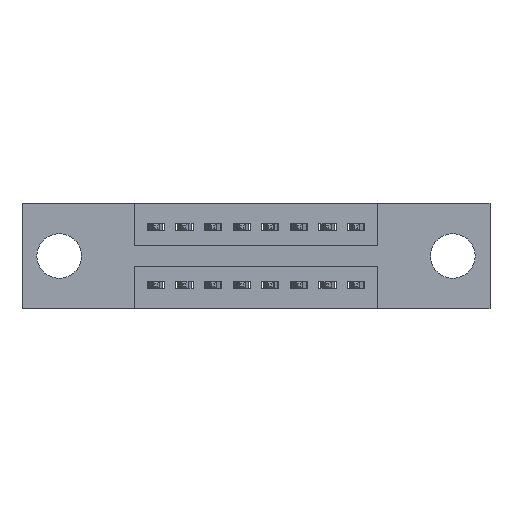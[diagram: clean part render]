
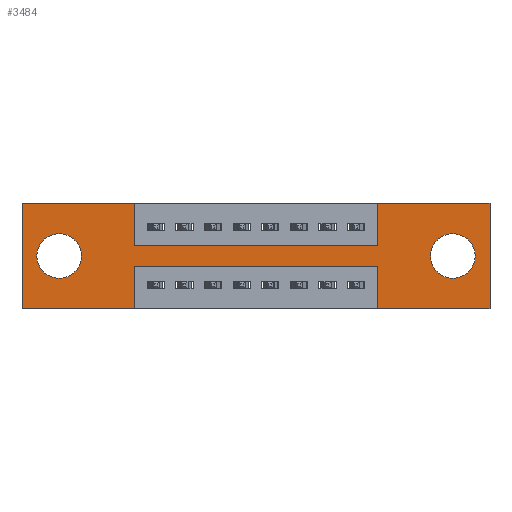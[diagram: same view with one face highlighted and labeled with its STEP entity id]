
A CAD part, front view. The second image highlights one B-rep face of the part: STEP entity #3484.
In plain terms, the highlighted planar face has unit normal (0, -1, 0).
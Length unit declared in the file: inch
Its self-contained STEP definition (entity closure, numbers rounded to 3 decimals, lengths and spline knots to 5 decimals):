
#56 = VERTEX_POINT ( 'NONE', #6474 ) ;
#128 = LINE ( 'NONE', #3564, #10887 ) ;
#141 = ORIENTED_EDGE ( 'NONE', *, *, #2143, .T. ) ;
#294 = CARTESIAN_POINT ( 'NONE',  ( 1.2425, 0., -0.37 ) ) ;
#381 = VERTEX_POINT ( 'NONE', #1865 ) ;
#614 = CARTESIAN_POINT ( 'NONE',  ( 0.13, 0., -0.185 ) ) ;
#624 = DIRECTION ( 'NONE',  ( 0., 1., 0. ) ) ;
#770 = ORIENTED_EDGE ( 'NONE', *, *, #3946, .T. ) ;
#771 = LINE ( 'NONE', #4481, #2104 ) ;
#1072 = VERTEX_POINT ( 'NONE', #7731 ) ;
#1081 = AXIS2_PLACEMENT_3D ( 'NONE', #614, #1631, #11090 ) ;
#1167 = PLANE ( 'NONE',  #10337 ) ;
#1365 = VECTOR ( 'NONE', #10003, 39.37008 ) ;
#1389 = ORIENTED_EDGE ( 'NONE', *, *, #3904, .T. ) ;
#1414 = ORIENTED_EDGE ( 'NONE', *, *, #4028, .F. ) ;
#1590 = DIRECTION ( 'NONE',  ( 0., 1., 0. ) ) ;
#1601 = VECTOR ( 'NONE', #9488, 39.37008 ) ;
#1631 = DIRECTION ( 'NONE',  ( 0., 1., 0. ) ) ;
#1865 = CARTESIAN_POINT ( 'NONE',  ( 0.3925, 0., -0.22 ) ) ;
#1912 = CIRCLE ( 'NONE', #9963, 0.078 ) ;
#2054 = EDGE_CURVE ( 'NONE', #2302, #4044, #771, .T. ) ;
#2103 = AXIS2_PLACEMENT_3D ( 'NONE', #3262, #624, #6704 ) ;
#2104 = VECTOR ( 'NONE', #9747, 39.37008 ) ;
#2143 = EDGE_CURVE ( 'NONE', #4229, #1072, #1912, .T. ) ;
#2271 = LINE ( 'NONE', #6739, #10328 ) ;
#2286 = VECTOR ( 'NONE', #9375, 39.37008 ) ;
#2302 = VERTEX_POINT ( 'NONE', #9396 ) ;
#2312 = VERTEX_POINT ( 'NONE', #2362 ) ;
#2362 = CARTESIAN_POINT ( 'NONE',  ( 1.2425, 0., -0.15 ) ) ;
#2506 = EDGE_CURVE ( 'NONE', #9969, #2302, #128, .T. ) ;
#2737 = EDGE_LOOP ( 'NONE', ( #770, #8006 ) ) ;
#2803 = DIRECTION ( 'NONE',  ( 0., 0., -1. ) ) ;
#2893 = DIRECTION ( 'NONE',  ( 0., 0., -1. ) ) ;
#2895 = CARTESIAN_POINT ( 'NONE',  ( 0., 0., -0.37 ) ) ;
#3186 = ORIENTED_EDGE ( 'NONE', *, *, #4300, .F. ) ;
#3262 = CARTESIAN_POINT ( 'NONE',  ( 1.505, 0., -0.185 ) ) ;
#3317 = LINE ( 'NONE', #9314, #1601 ) ;
#3342 = DIRECTION ( 'NONE',  ( 0., 0., 1. ) ) ;
#3469 = LINE ( 'NONE', #5194, #10599 ) ;
#3484 = ADVANCED_FACE ( 'NONE', ( #5645, #8948, #8096 ), #1167, .T. ) ;
#3541 = LINE ( 'NONE', #4501, #6205 ) ;
#3564 = CARTESIAN_POINT ( 'NONE',  ( 0., 0., 0. ) ) ;
#3904 = EDGE_CURVE ( 'NONE', #1072, #4229, #10319, .T. ) ;
#3946 = EDGE_CURVE ( 'NONE', #6277, #10006, #5950, .T. ) ;
#4001 = CARTESIAN_POINT ( 'NONE',  ( 0.3925, 0., -0.37 ) ) ;
#4028 = EDGE_CURVE ( 'NONE', #6402, #381, #8467, .T. ) ;
#4044 = VERTEX_POINT ( 'NONE', #5149 ) ;
#4045 = DIRECTION ( 'NONE',  ( 0., 0., 1. ) ) ;
#4150 = DIRECTION ( 'NONE',  ( 0., 0., -1. ) ) ;
#4229 = VERTEX_POINT ( 'NONE', #8909 ) ;
#4300 = EDGE_CURVE ( 'NONE', #4044, #2312, #5488, .T. ) ;
#4401 = CARTESIAN_POINT ( 'NONE',  ( 0., 0., 0. ) ) ;
#4447 = EDGE_CURVE ( 'NONE', #381, #7881, #2271, .T. ) ;
#4481 = CARTESIAN_POINT ( 'NONE',  ( 0.3925, 0., 0. ) ) ;
#4501 = CARTESIAN_POINT ( 'NONE',  ( 1.635, 0., 0. ) ) ;
#4542 = CARTESIAN_POINT ( 'NONE',  ( 0., 0., 0. ) ) ;
#4575 = EDGE_CURVE ( 'NONE', #9108, #10489, #7134, .T. ) ;
#4596 = DIRECTION ( 'NONE',  ( 0., 0., -1. ) ) ;
#4633 = DIRECTION ( 'NONE',  ( 0., 0., 1. ) ) ;
#4655 = CARTESIAN_POINT ( 'NONE',  ( 1.505, 0., -0.185 ) ) ;
#4678 = VERTEX_POINT ( 'NONE', #8953 ) ;
#4732 = EDGE_LOOP ( 'NONE', ( #6372, #1414, #6492, #9165, #5458, #6764, #5681, #3186, #6796, #7961, #10584, #8187 ) ) ;
#4871 = EDGE_CURVE ( 'NONE', #56, #9969, #5334, .T. ) ;
#5013 = EDGE_CURVE ( 'NONE', #2312, #9108, #8306, .T. ) ;
#5118 = CARTESIAN_POINT ( 'NONE',  ( 0.13, 0., -0.107 ) ) ;
#5149 = CARTESIAN_POINT ( 'NONE',  ( 0.3925, 0., -0.15 ) ) ;
#5194 = CARTESIAN_POINT ( 'NONE',  ( 0., 0., -0.37 ) ) ;
#5227 = DIRECTION ( 'NONE',  ( 1., 0., 0. ) ) ;
#5232 = EDGE_CURVE ( 'NONE', #7881, #56, #3317, .T. ) ;
#5244 = CARTESIAN_POINT ( 'NONE',  ( 0., 0., 0. ) ) ;
#5334 = LINE ( 'NONE', #4401, #10747 ) ;
#5394 = EDGE_CURVE ( 'NONE', #10489, #4678, #3541, .T. ) ;
#5458 = ORIENTED_EDGE ( 'NONE', *, *, #5394, .F. ) ;
#5488 = LINE ( 'NONE', #9948, #1365 ) ;
#5645 = FACE_BOUND ( 'NONE', #9256, .T. ) ;
#5681 = ORIENTED_EDGE ( 'NONE', *, *, #5013, .F. ) ;
#5902 = CARTESIAN_POINT ( 'NONE',  ( 0.3925, 0., -0.22 ) ) ;
#5950 = CIRCLE ( 'NONE', #10133, 0.078 ) ;
#6032 = CIRCLE ( 'NONE', #1081, 0.078 ) ;
#6205 = VECTOR ( 'NONE', #2803, 39.37008 ) ;
#6277 = VERTEX_POINT ( 'NONE', #5118 ) ;
#6372 = ORIENTED_EDGE ( 'NONE', *, *, #4447, .F. ) ;
#6402 = VERTEX_POINT ( 'NONE', #10714 ) ;
#6474 = CARTESIAN_POINT ( 'NONE',  ( 0., 0., -0.37 ) ) ;
#6492 = ORIENTED_EDGE ( 'NONE', *, *, #6970, .F. ) ;
#6595 = CARTESIAN_POINT ( 'NONE',  ( 1.2425, 0., 0. ) ) ;
#6691 = VECTOR ( 'NONE', #10438, 39.37008 ) ;
#6704 = DIRECTION ( 'NONE',  ( 0., 0., -1. ) ) ;
#6739 = CARTESIAN_POINT ( 'NONE',  ( 0.3925, 0., -0.37 ) ) ;
#6764 = ORIENTED_EDGE ( 'NONE', *, *, #4575, .F. ) ;
#6796 = ORIENTED_EDGE ( 'NONE', *, *, #2054, .F. ) ;
#6970 = EDGE_CURVE ( 'NONE', #9048, #6402, #10281, .T. ) ;
#7134 = LINE ( 'NONE', #5244, #6691 ) ;
#7465 = CARTESIAN_POINT ( 'NONE',  ( 1.635, 0., 0. ) ) ;
#7502 = CARTESIAN_POINT ( 'NONE',  ( 0.13, 0., -0.185 ) ) ;
#7731 = CARTESIAN_POINT ( 'NONE',  ( 1.505, 0., -0.107 ) ) ;
#7874 = DIRECTION ( 'NONE',  ( -1., 0., 0. ) ) ;
#7881 = VERTEX_POINT ( 'NONE', #4001 ) ;
#7961 = ORIENTED_EDGE ( 'NONE', *, *, #2506, .F. ) ;
#8006 = ORIENTED_EDGE ( 'NONE', *, *, #9620, .T. ) ;
#8096 = FACE_OUTER_BOUND ( 'NONE', #4732, .T. ) ;
#8106 = CARTESIAN_POINT ( 'NONE',  ( 0.13, 0., -0.263 ) ) ;
#8187 = ORIENTED_EDGE ( 'NONE', *, *, #5232, .F. ) ;
#8306 = LINE ( 'NONE', #9907, #8372 ) ;
#8372 = VECTOR ( 'NONE', #4633, 39.37008 ) ;
#8467 = LINE ( 'NONE', #5902, #2286 ) ;
#8909 = CARTESIAN_POINT ( 'NONE',  ( 1.505, 0., -0.263 ) ) ;
#8948 = FACE_BOUND ( 'NONE', #2737, .T. ) ;
#8953 = CARTESIAN_POINT ( 'NONE',  ( 1.635, 0., -0.37 ) ) ;
#9008 = DIRECTION ( 'NONE',  ( 0., -1., 0. ) ) ;
#9048 = VERTEX_POINT ( 'NONE', #294 ) ;
#9108 = VERTEX_POINT ( 'NONE', #6595 ) ;
#9141 = VECTOR ( 'NONE', #4045, 39.37008 ) ;
#9165 = ORIENTED_EDGE ( 'NONE', *, *, #9833, .F. ) ;
#9256 = EDGE_LOOP ( 'NONE', ( #1389, #141 ) ) ;
#9314 = CARTESIAN_POINT ( 'NONE',  ( 0., 0., -0.37 ) ) ;
#9375 = DIRECTION ( 'NONE',  ( -1., 0., 0. ) ) ;
#9396 = CARTESIAN_POINT ( 'NONE',  ( 0.3925, 0., 0. ) ) ;
#9423 = CARTESIAN_POINT ( 'NONE',  ( 1.2425, 0., -0.37 ) ) ;
#9488 = DIRECTION ( 'NONE',  ( -1., 0., 0. ) ) ;
#9620 = EDGE_CURVE ( 'NONE', #10006, #6277, #6032, .T. ) ;
#9747 = DIRECTION ( 'NONE',  ( 0., 0., -1. ) ) ;
#9833 = EDGE_CURVE ( 'NONE', #4678, #9048, #3469, .T. ) ;
#9907 = CARTESIAN_POINT ( 'NONE',  ( 1.2425, 0., 0. ) ) ;
#9948 = CARTESIAN_POINT ( 'NONE',  ( 0.3925, 0., -0.15 ) ) ;
#9963 = AXIS2_PLACEMENT_3D ( 'NONE', #4655, #10720, #2893 ) ;
#9969 = VERTEX_POINT ( 'NONE', #4542 ) ;
#10003 = DIRECTION ( 'NONE',  ( 1., 0., 0. ) ) ;
#10006 = VERTEX_POINT ( 'NONE', #8106 ) ;
#10133 = AXIS2_PLACEMENT_3D ( 'NONE', #7502, #1590, #10987 ) ;
#10281 = LINE ( 'NONE', #9423, #9141 ) ;
#10319 = CIRCLE ( 'NONE', #2103, 0.078 ) ;
#10328 = VECTOR ( 'NONE', #4150, 39.37008 ) ;
#10337 = AXIS2_PLACEMENT_3D ( 'NONE', #2895, #9008, #4596 ) ;
#10438 = DIRECTION ( 'NONE',  ( 1., 0., 0. ) ) ;
#10489 = VERTEX_POINT ( 'NONE', #7465 ) ;
#10584 = ORIENTED_EDGE ( 'NONE', *, *, #4871, .F. ) ;
#10599 = VECTOR ( 'NONE', #7874, 39.37008 ) ;
#10714 = CARTESIAN_POINT ( 'NONE',  ( 1.2425, 0., -0.22 ) ) ;
#10720 = DIRECTION ( 'NONE',  ( 0., 1., 0. ) ) ;
#10747 = VECTOR ( 'NONE', #3342, 39.37008 ) ;
#10887 = VECTOR ( 'NONE', #5227, 39.37008 ) ;
#10987 = DIRECTION ( 'NONE',  ( 0., 0., 1. ) ) ;
#11090 = DIRECTION ( 'NONE',  ( 0., 0., 1. ) ) ;
